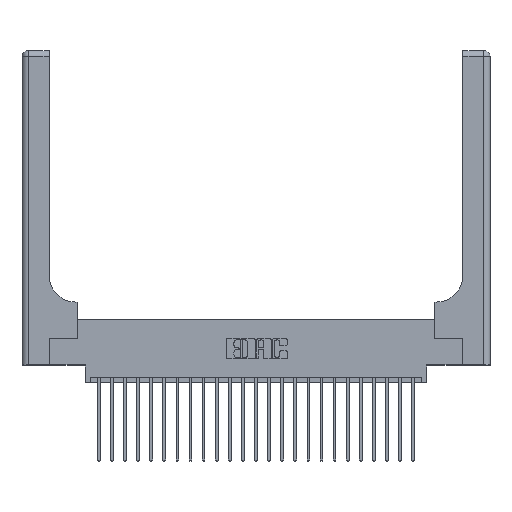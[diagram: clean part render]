
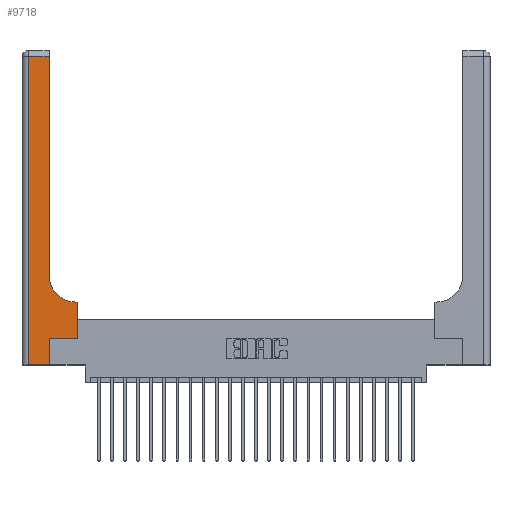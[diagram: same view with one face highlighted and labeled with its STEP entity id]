
A CAD part, top view. The second image highlights one B-rep face of the part: STEP entity #9718.
In plain terms, the highlighted planar face has unit normal (0, 0, 1).
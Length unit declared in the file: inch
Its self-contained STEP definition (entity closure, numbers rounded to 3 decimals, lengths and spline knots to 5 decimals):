
#1894 = ORIENTED_EDGE ( 'NONE', *, *, #19381, .T. ) ;
#2014 = EDGE_CURVE ( 'NONE', #3441, #17804, #19472, .T. ) ;
#2107 = EDGE_CURVE ( 'NONE', #10126, #20658, #10044, .T. ) ;
#2479 = VECTOR ( 'NONE', #21603, 39.37008 ) ;
#2667 = EDGE_CURVE ( 'NONE', #17804, #10126, #18154, .T. ) ;
#2727 = DIRECTION ( 'NONE',  ( 0., 0., -1. ) ) ;
#2968 = PLANE ( 'NONE',  #19560 ) ;
#3003 = VECTOR ( 'NONE', #14189, 39.37008 ) ;
#3220 = DIRECTION ( 'NONE',  ( 0., 1., 0. ) ) ;
#3441 = VERTEX_POINT ( 'NONE', #13870 ) ;
#4005 = CARTESIAN_POINT ( 'NONE',  ( 0.51, 0.85, 0.37 ) ) ;
#4328 = ORIENTED_EDGE ( 'NONE', *, *, #5015, .T. ) ;
#4398 = CARTESIAN_POINT ( 'NONE',  ( 0.265, 0.25, 0.37 ) ) ;
#4501 = AXIS2_PLACEMENT_3D ( 'NONE', #4005, #20768, #15234 ) ;
#4971 = CARTESIAN_POINT ( 'NONE',  ( 0.265, 0.25, 0.37 ) ) ;
#5015 = EDGE_CURVE ( 'NONE', #9352, #11909, #19753, .T. ) ;
#5059 = CARTESIAN_POINT ( 'NONE',  ( 0.26, 3., 0.37 ) ) ;
#5478 = ORIENTED_EDGE ( 'NONE', *, *, #2014, .T. ) ;
#5511 = VECTOR ( 'NONE', #5962, 39.37008 ) ;
#5644 = CARTESIAN_POINT ( 'NONE',  ( 0.26, 2.94, 0.37 ) ) ;
#5685 = DIRECTION ( 'NONE',  ( 0., -1., 0. ) ) ;
#5699 = ORIENTED_EDGE ( 'NONE', *, *, #7301, .T. ) ;
#5962 = DIRECTION ( 'NONE',  ( -1., 0., 0. ) ) ;
#6071 = VERTEX_POINT ( 'NONE', #20370 ) ;
#6183 = LINE ( 'NONE', #13842, #8655 ) ;
#7301 = EDGE_CURVE ( 'NONE', #20658, #10980, #20864, .T. ) ;
#8276 = VECTOR ( 'NONE', #10295, 39.37008 ) ;
#8515 = ORIENTED_EDGE ( 'NONE', *, *, #16515, .T. ) ;
#8655 = VECTOR ( 'NONE', #12003, 39.37008 ) ;
#9054 = CARTESIAN_POINT ( 'NONE',  ( 0.06, 2.94, 0.37 ) ) ;
#9130 = DIRECTION ( 'NONE',  ( 0., 1., 0. ) ) ;
#9352 = VERTEX_POINT ( 'NONE', #20125 ) ;
#9718 = ADVANCED_FACE ( 'NONE', ( #23570 ), #2968, .F. ) ;
#10044 = LINE ( 'NONE', #15843, #5511 ) ;
#10126 = VERTEX_POINT ( 'NONE', #5644 ) ;
#10295 = DIRECTION ( 'NONE',  ( 1., 0., 0. ) ) ;
#10980 = VERTEX_POINT ( 'NONE', #19633 ) ;
#11909 = VERTEX_POINT ( 'NONE', #4398 ) ;
#11999 = CARTESIAN_POINT ( 'NONE',  ( 0.26, 0.6, 0.37 ) ) ;
#12003 = DIRECTION ( 'NONE',  ( 1., 0., 0. ) ) ;
#12563 = VECTOR ( 'NONE', #9130, 39.37008 ) ;
#13092 = CARTESIAN_POINT ( 'NONE',  ( 0.528, 0.25, 0.37 ) ) ;
#13202 = CARTESIAN_POINT ( 'NONE',  ( 0.528, 0.6, 0.37 ) ) ;
#13544 = EDGE_CURVE ( 'NONE', #6071, #23114, #15311, .T. ) ;
#13838 = LINE ( 'NONE', #11999, #2479 ) ;
#13842 = CARTESIAN_POINT ( 'NONE',  ( 0., 0., 0.37 ) ) ;
#13870 = CARTESIAN_POINT ( 'NONE',  ( 0.51, 0.6, 0.37 ) ) ;
#14036 = EDGE_LOOP ( 'NONE', ( #16553, #20296, #5699, #20277, #4328, #8515, #24346, #1894, #5478 ) ) ;
#14189 = DIRECTION ( 'NONE',  ( 0., 1., 0. ) ) ;
#15234 = DIRECTION ( 'NONE',  ( 1., 0., 0. ) ) ;
#15311 = LINE ( 'NONE', #13092, #12563 ) ;
#15843 = CARTESIAN_POINT ( 'NONE',  ( 0., 2.94, 0.37 ) ) ;
#16515 = EDGE_CURVE ( 'NONE', #11909, #6071, #21866, .T. ) ;
#16553 = ORIENTED_EDGE ( 'NONE', *, *, #2667, .T. ) ;
#16894 = VECTOR ( 'NONE', #3220, 39.37008 ) ;
#17804 = VERTEX_POINT ( 'NONE', #19900 ) ;
#18135 = CARTESIAN_POINT ( 'NONE',  ( 0., 3., 0.37 ) ) ;
#18154 = LINE ( 'NONE', #5059, #16894 ) ;
#19381 = EDGE_CURVE ( 'NONE', #23114, #3441, #13838, .T. ) ;
#19472 = CIRCLE ( 'NONE', #4501, 0.25 ) ;
#19560 = AXIS2_PLACEMENT_3D ( 'NONE', #18135, #2727, #23454 ) ;
#19631 = VECTOR ( 'NONE', #5685, 39.37008 ) ;
#19633 = CARTESIAN_POINT ( 'NONE',  ( 0.06, 0., 0.37 ) ) ;
#19753 = LINE ( 'NONE', #21477, #3003 ) ;
#19900 = CARTESIAN_POINT ( 'NONE',  ( 0.26, 0.85, 0.37 ) ) ;
#20125 = CARTESIAN_POINT ( 'NONE',  ( 0.265, 0., 0.37 ) ) ;
#20277 = ORIENTED_EDGE ( 'NONE', *, *, #22893, .T. ) ;
#20296 = ORIENTED_EDGE ( 'NONE', *, *, #2107, .T. ) ;
#20370 = CARTESIAN_POINT ( 'NONE',  ( 0.528, 0.25, 0.37 ) ) ;
#20658 = VERTEX_POINT ( 'NONE', #9054 ) ;
#20768 = DIRECTION ( 'NONE',  ( 0., 0., -1. ) ) ;
#20864 = LINE ( 'NONE', #24334, #19631 ) ;
#21477 = CARTESIAN_POINT ( 'NONE',  ( 0.265, 0., 0.37 ) ) ;
#21603 = DIRECTION ( 'NONE',  ( -1., 0., 0. ) ) ;
#21866 = LINE ( 'NONE', #4971, #8276 ) ;
#22893 = EDGE_CURVE ( 'NONE', #10980, #9352, #6183, .T. ) ;
#23114 = VERTEX_POINT ( 'NONE', #13202 ) ;
#23454 = DIRECTION ( 'NONE',  ( -1., 0., 0. ) ) ;
#23570 = FACE_OUTER_BOUND ( 'NONE', #14036, .T. ) ;
#24334 = CARTESIAN_POINT ( 'NONE',  ( 0.06, 3., 0.37 ) ) ;
#24346 = ORIENTED_EDGE ( 'NONE', *, *, #13544, .T. ) ;
